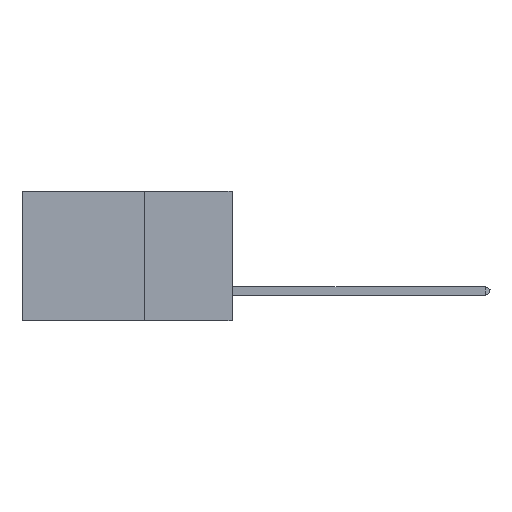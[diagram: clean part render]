
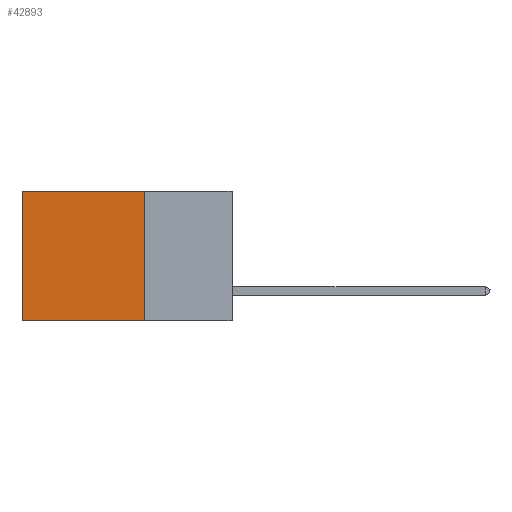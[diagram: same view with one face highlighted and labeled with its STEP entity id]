
A CAD part, left-side view. The second image highlights one B-rep face of the part: STEP entity #42893.
In plain terms, the highlighted planar face has unit normal (-1, 0, 0).
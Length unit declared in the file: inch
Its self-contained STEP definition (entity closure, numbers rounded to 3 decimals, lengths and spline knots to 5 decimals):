
#724 = DIRECTION ( 'NONE',  ( 0., 0., -1. ) ) ;
#3195 = VECTOR ( 'NONE', #37135, 39.37008 ) ;
#3750 = ORIENTED_EDGE ( 'NONE', *, *, #19717, .F. ) ;
#4305 = CARTESIAN_POINT ( 'NONE',  ( 0.2875, 0.25, 0. ) ) ;
#4666 = AXIS2_PLACEMENT_3D ( 'NONE', #4305, #14526, #21147 ) ;
#4786 = EDGE_LOOP ( 'NONE', ( #15099, #43457, #3750, #36269 ) ) ;
#5711 = VECTOR ( 'NONE', #724, 39.37008 ) ;
#6027 = CARTESIAN_POINT ( 'NONE',  ( 0.2875, 0.25, 0. ) ) ;
#8122 = CARTESIAN_POINT ( 'NONE',  ( 0.2875, 0.25, -0.37 ) ) ;
#8342 = LINE ( 'NONE', #34281, #5711 ) ;
#10152 = VERTEX_POINT ( 'NONE', #24549 ) ;
#14526 = DIRECTION ( 'NONE',  ( 1., 0., 0. ) ) ;
#14749 = DIRECTION ( 'NONE',  ( 0., 0., -1. ) ) ;
#14858 = FACE_OUTER_BOUND ( 'NONE', #4786, .T. ) ;
#15099 = ORIENTED_EDGE ( 'NONE', *, *, #19421, .T. ) ;
#16455 = VECTOR ( 'NONE', #14749, 39.37008 ) ;
#16946 = LINE ( 'NONE', #17612, #29846 ) ;
#17612 = CARTESIAN_POINT ( 'NONE',  ( 0.2875, 0.25, -0.37 ) ) ;
#17719 = VERTEX_POINT ( 'NONE', #8122 ) ;
#19205 = VERTEX_POINT ( 'NONE', #35271 ) ;
#19421 = EDGE_CURVE ( 'NONE', #29270, #10152, #8342, .T. ) ;
#19717 = EDGE_CURVE ( 'NONE', #19205, #17719, #26667, .T. ) ;
#21147 = DIRECTION ( 'NONE',  ( 0., 0., -1. ) ) ;
#21341 = DIRECTION ( 'NONE',  ( 0., 1., 0. ) ) ;
#23212 = CARTESIAN_POINT ( 'NONE',  ( 0.2875, 0.6, 0. ) ) ;
#24549 = CARTESIAN_POINT ( 'NONE',  ( 0.2875, 0.6, -0.37 ) ) ;
#26383 = EDGE_CURVE ( 'NONE', #19205, #29270, #40801, .T. ) ;
#26667 = LINE ( 'NONE', #28259, #16455 ) ;
#28194 = PLANE ( 'NONE',  #4666 ) ;
#28259 = CARTESIAN_POINT ( 'NONE',  ( 0.2875, 0.25, 0. ) ) ;
#29270 = VERTEX_POINT ( 'NONE', #23212 ) ;
#29846 = VECTOR ( 'NONE', #21341, 39.37008 ) ;
#34281 = CARTESIAN_POINT ( 'NONE',  ( 0.2875, 0.6, 0. ) ) ;
#35271 = CARTESIAN_POINT ( 'NONE',  ( 0.2875, 0.25, 0. ) ) ;
#36269 = ORIENTED_EDGE ( 'NONE', *, *, #26383, .T. ) ;
#37135 = DIRECTION ( 'NONE',  ( 0., 1., 0. ) ) ;
#40801 = LINE ( 'NONE', #6027, #3195 ) ;
#42893 = ADVANCED_FACE ( 'NONE', ( #14858 ), #28194, .F. ) ;
#43457 = ORIENTED_EDGE ( 'NONE', *, *, #44139, .F. ) ;
#44139 = EDGE_CURVE ( 'NONE', #17719, #10152, #16946, .T. ) ;
